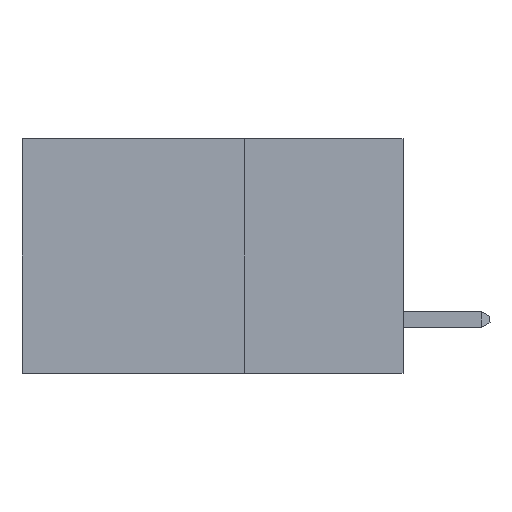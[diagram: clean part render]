
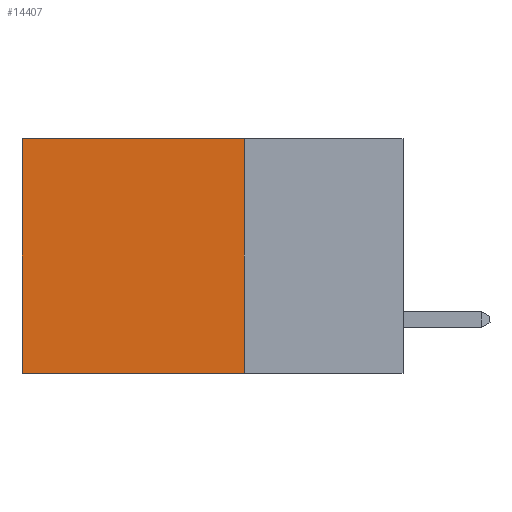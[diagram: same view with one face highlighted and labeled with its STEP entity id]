
A CAD part, left-side view. The second image highlights one B-rep face of the part: STEP entity #14407.
In plain terms, the highlighted planar face has unit normal (-1, 0, 0).
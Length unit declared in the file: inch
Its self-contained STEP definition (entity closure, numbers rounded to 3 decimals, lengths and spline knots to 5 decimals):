
#864 = ORIENTED_EDGE ( 'NONE', *, *, #4109, .F. ) ;
#1062 = DIRECTION ( 'NONE',  ( 0., 1., 0. ) ) ;
#1101 = DIRECTION ( 'NONE',  ( 0., 0., -1. ) ) ;
#1589 = CARTESIAN_POINT ( 'NONE',  ( 0.2875, 0.25, -0.37 ) ) ;
#2829 = LINE ( 'NONE', #15436, #3585 ) ;
#3469 = ORIENTED_EDGE ( 'NONE', *, *, #11815, .F. ) ;
#3585 = VECTOR ( 'NONE', #1062, 39.37008 ) ;
#4036 = ORIENTED_EDGE ( 'NONE', *, *, #17604, .T. ) ;
#4109 = EDGE_CURVE ( 'NONE', #24631, #11338, #25659, .T. ) ;
#4111 = DIRECTION ( 'NONE',  ( 0., 0., -1. ) ) ;
#7075 = VECTOR ( 'NONE', #15391, 39.37008 ) ;
#9776 = EDGE_LOOP ( 'NONE', ( #4036, #3469, #864, #18088 ) ) ;
#10360 = AXIS2_PLACEMENT_3D ( 'NONE', #30309, #18445, #4111 ) ;
#11338 = VERTEX_POINT ( 'NONE', #1589 ) ;
#11815 = EDGE_CURVE ( 'NONE', #11338, #20506, #19763, .T. ) ;
#12106 = CARTESIAN_POINT ( 'NONE',  ( 0.2875, 0.25, 0. ) ) ;
#12205 = VECTOR ( 'NONE', #1101, 39.37008 ) ;
#13100 = CARTESIAN_POINT ( 'NONE',  ( 0.2875, 0.6, -0.37 ) ) ;
#13715 = EDGE_CURVE ( 'NONE', #24631, #14475, #2829, .T. ) ;
#14407 = ADVANCED_FACE ( 'NONE', ( #24137 ), #16046, .F. ) ;
#14475 = VERTEX_POINT ( 'NONE', #20841 ) ;
#15391 = DIRECTION ( 'NONE',  ( 0., 1., 0. ) ) ;
#15436 = CARTESIAN_POINT ( 'NONE',  ( 0.2875, 0.25, 0. ) ) ;
#16046 = PLANE ( 'NONE',  #10360 ) ;
#16612 = CARTESIAN_POINT ( 'NONE',  ( 0.2875, 0.6, 0. ) ) ;
#17604 = EDGE_CURVE ( 'NONE', #14475, #20506, #19955, .T. ) ;
#17818 = CARTESIAN_POINT ( 'NONE',  ( 0.2875, 0.25, -0.37 ) ) ;
#18088 = ORIENTED_EDGE ( 'NONE', *, *, #13715, .T. ) ;
#18445 = DIRECTION ( 'NONE',  ( 1., 0., 0. ) ) ;
#18476 = VECTOR ( 'NONE', #26129, 39.37008 ) ;
#19763 = LINE ( 'NONE', #17818, #7075 ) ;
#19955 = LINE ( 'NONE', #16612, #18476 ) ;
#20506 = VERTEX_POINT ( 'NONE', #13100 ) ;
#20841 = CARTESIAN_POINT ( 'NONE',  ( 0.2875, 0.6, 0. ) ) ;
#24137 = FACE_OUTER_BOUND ( 'NONE', #9776, .T. ) ;
#24631 = VERTEX_POINT ( 'NONE', #12106 ) ;
#25136 = CARTESIAN_POINT ( 'NONE',  ( 0.2875, 0.25, 0. ) ) ;
#25659 = LINE ( 'NONE', #25136, #12205 ) ;
#26129 = DIRECTION ( 'NONE',  ( 0., 0., -1. ) ) ;
#30309 = CARTESIAN_POINT ( 'NONE',  ( 0.2875, 0.25, 0. ) ) ;
